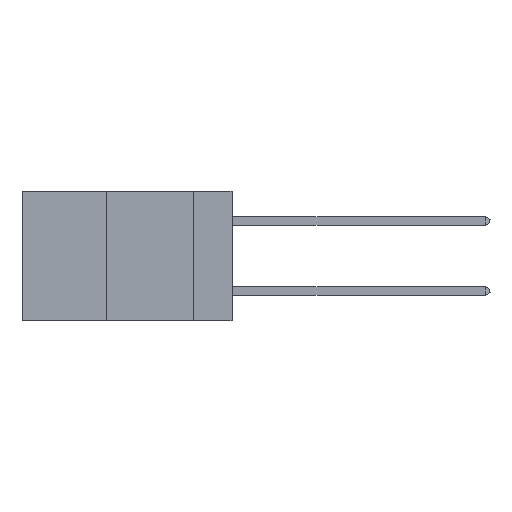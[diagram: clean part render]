
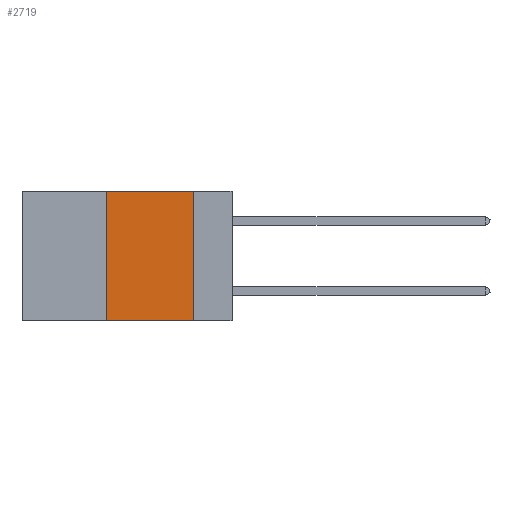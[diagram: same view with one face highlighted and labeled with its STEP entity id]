
A CAD part, left-side view. The second image highlights one B-rep face of the part: STEP entity #2719.
In plain terms, the highlighted planar face has unit normal (-1, 0, 0).
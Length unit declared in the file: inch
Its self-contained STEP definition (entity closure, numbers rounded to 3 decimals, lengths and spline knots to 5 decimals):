
#509 = VECTOR ( 'NONE', #32572, 39.37008 ) ;
#529 = LINE ( 'NONE', #19062, #3098 ) ;
#1949 = VECTOR ( 'NONE', #19090, 39.37008 ) ;
#2719 = ADVANCED_FACE ( 'NONE', ( #9056 ), #21562, .F. ) ;
#3098 = VECTOR ( 'NONE', #13640, 39.37008 ) ;
#5112 = VERTEX_POINT ( 'NONE', #28023 ) ;
#5354 = EDGE_CURVE ( 'NONE', #31227, #23021, #9273, .T. ) ;
#9056 = FACE_OUTER_BOUND ( 'NONE', #18899, .T. ) ;
#9273 = LINE ( 'NONE', #10519, #1949 ) ;
#9573 = VERTEX_POINT ( 'NONE', #28752 ) ;
#10076 = CARTESIAN_POINT ( 'NONE',  ( 0., 0.11, -0.37 ) ) ;
#10519 = CARTESIAN_POINT ( 'NONE',  ( 0., 0.6, -0.37 ) ) ;
#13246 = DIRECTION ( 'NONE',  ( 1., 0., 0. ) ) ;
#13301 = CARTESIAN_POINT ( 'NONE',  ( 0., 0.6, 0. ) ) ;
#13640 = DIRECTION ( 'NONE',  ( 0., 0., -1. ) ) ;
#14654 = AXIS2_PLACEMENT_3D ( 'NONE', #35219, #13246, #32761 ) ;
#15226 = EDGE_CURVE ( 'NONE', #5112, #9573, #19502, .T. ) ;
#17779 = LINE ( 'NONE', #30139, #29409 ) ;
#18899 = EDGE_LOOP ( 'NONE', ( #31280, #24128, #29013, #26744 ) ) ;
#19062 = CARTESIAN_POINT ( 'NONE',  ( 0., 0.11, 0. ) ) ;
#19090 = DIRECTION ( 'NONE',  ( 0., -1., 0. ) ) ;
#19502 = LINE ( 'NONE', #13301, #509 ) ;
#21562 = PLANE ( 'NONE',  #14654 ) ;
#21960 = DIRECTION ( 'NONE',  ( 0., 0., 1. ) ) ;
#23021 = VERTEX_POINT ( 'NONE', #10076 ) ;
#24128 = ORIENTED_EDGE ( 'NONE', *, *, #15226, .F. ) ;
#26744 = ORIENTED_EDGE ( 'NONE', *, *, #5354, .T. ) ;
#28023 = CARTESIAN_POINT ( 'NONE',  ( 0., 0.36, 0. ) ) ;
#28752 = CARTESIAN_POINT ( 'NONE',  ( 0., 0.11, 0. ) ) ;
#29013 = ORIENTED_EDGE ( 'NONE', *, *, #30367, .F. ) ;
#29409 = VECTOR ( 'NONE', #21960, 39.37008 ) ;
#30139 = CARTESIAN_POINT ( 'NONE',  ( 0., 0.36, 0. ) ) ;
#30367 = EDGE_CURVE ( 'NONE', #31227, #5112, #17779, .T. ) ;
#30404 = EDGE_CURVE ( 'NONE', #9573, #23021, #529, .T. ) ;
#31227 = VERTEX_POINT ( 'NONE', #33500 ) ;
#31280 = ORIENTED_EDGE ( 'NONE', *, *, #30404, .F. ) ;
#32572 = DIRECTION ( 'NONE',  ( 0., -1., 0. ) ) ;
#32761 = DIRECTION ( 'NONE',  ( 0., 0., -1. ) ) ;
#33500 = CARTESIAN_POINT ( 'NONE',  ( 0., 0.36, -0.37 ) ) ;
#35219 = CARTESIAN_POINT ( 'NONE',  ( 0., 0.6, 0. ) ) ;
